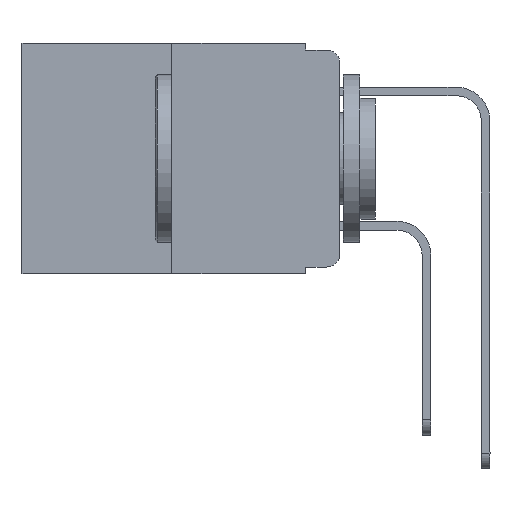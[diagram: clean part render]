
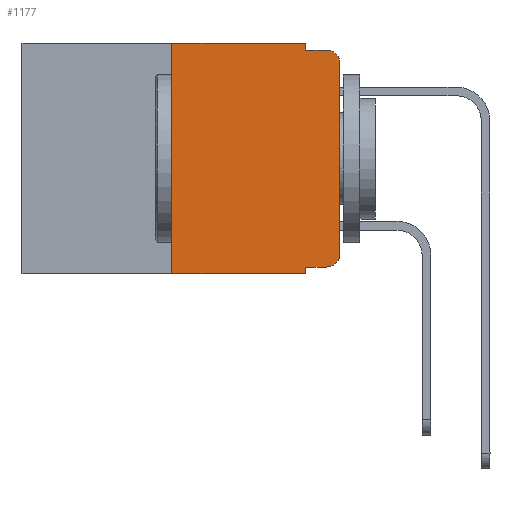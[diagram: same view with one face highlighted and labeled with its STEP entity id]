
A CAD part, left-side view. The second image highlights one B-rep face of the part: STEP entity #1177.
In plain terms, the highlighted planar face has unit normal (-1, 0, 0).
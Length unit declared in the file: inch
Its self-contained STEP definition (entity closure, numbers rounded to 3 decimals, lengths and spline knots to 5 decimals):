
#102 = EDGE_CURVE ( 'NONE', #10034, #8125, #7041, .T. ) ;
#169 = VECTOR ( 'NONE', #8905, 39.37008 ) ;
#408 = LINE ( 'NONE', #1333, #6631 ) ;
#523 = VECTOR ( 'NONE', #4066, 39.37008 ) ;
#565 = CARTESIAN_POINT ( 'NONE',  ( 0., 0.25, 0. ) ) ;
#645 = LINE ( 'NONE', #7770, #7120 ) ;
#703 = LINE ( 'NONE', #6839, #169 ) ;
#1177 = ADVANCED_FACE ( 'NONE', ( #7506 ), #9507, .F. ) ;
#1267 = CARTESIAN_POINT ( 'NONE',  ( 0., 0.02, -0.313 ) ) ;
#1333 = CARTESIAN_POINT ( 'NONE',  ( 0., 0.051, -0.333 ) ) ;
#1868 = DIRECTION ( 'NONE',  ( 0., 0., -1. ) ) ;
#2195 = AXIS2_PLACEMENT_3D ( 'NONE', #5825, #8612, #1868 ) ;
#2274 = VERTEX_POINT ( 'NONE', #9673 ) ;
#2414 = DIRECTION ( 'NONE',  ( 0., -1., 0. ) ) ;
#2418 = VECTOR ( 'NONE', #7237, 39.37008 ) ;
#2542 = CARTESIAN_POINT ( 'NONE',  ( 0., 0.25, -0.343 ) ) ;
#2949 = EDGE_CURVE ( 'NONE', #4676, #5879, #6572, .T. ) ;
#3016 = VERTEX_POINT ( 'NONE', #565 ) ;
#3075 = CARTESIAN_POINT ( 'NONE',  ( 0., 0.02, -0.333 ) ) ;
#3204 = DIRECTION ( 'NONE',  ( 0., 0., -1. ) ) ;
#3265 = ORIENTED_EDGE ( 'NONE', *, *, #8750, .T. ) ;
#3638 = DIRECTION ( 'NONE',  ( -1., 0., 0. ) ) ;
#3937 = CARTESIAN_POINT ( 'NONE',  ( 0., 0., 0. ) ) ;
#3944 = ORIENTED_EDGE ( 'NONE', *, *, #8931, .F. ) ;
#4066 = DIRECTION ( 'NONE',  ( 0., 0., 1. ) ) ;
#4118 = VERTEX_POINT ( 'NONE', #13077 ) ;
#4213 = LINE ( 'NONE', #7182, #4791 ) ;
#4479 = AXIS2_PLACEMENT_3D ( 'NONE', #11555, #5319, #10376 ) ;
#4546 = LINE ( 'NONE', #3937, #523 ) ;
#4676 = VERTEX_POINT ( 'NONE', #2542 ) ;
#4791 = VECTOR ( 'NONE', #8056, 39.37008 ) ;
#5319 = DIRECTION ( 'NONE',  ( 1., 0., 0. ) ) ;
#5446 = VECTOR ( 'NONE', #3204, 39.37008 ) ;
#5519 = VERTEX_POINT ( 'NONE', #9796 ) ;
#5686 = CARTESIAN_POINT ( 'NONE',  ( 0., 0., -0.313 ) ) ;
#5825 = CARTESIAN_POINT ( 'NONE',  ( 0., 0.02, -0.03 ) ) ;
#5879 = VERTEX_POINT ( 'NONE', #6442 ) ;
#5960 = VECTOR ( 'NONE', #2414, 39.37008 ) ;
#6274 = EDGE_LOOP ( 'NONE', ( #3265, #7491, #10293, #9197, #3944, #6538, #10992, #10276, #8016, #8421 ) ) ;
#6439 = LINE ( 'NONE', #9430, #5446 ) ;
#6442 = CARTESIAN_POINT ( 'NONE',  ( 0., 0.051, -0.343 ) ) ;
#6538 = ORIENTED_EDGE ( 'NONE', *, *, #12137, .F. ) ;
#6572 = LINE ( 'NONE', #9560, #5960 ) ;
#6631 = VECTOR ( 'NONE', #12517, 39.37008 ) ;
#6689 = EDGE_CURVE ( 'NONE', #2274, #11320, #408, .T. ) ;
#6839 = CARTESIAN_POINT ( 'NONE',  ( 0., 0.051, -0.01 ) ) ;
#6864 = EDGE_CURVE ( 'NONE', #11320, #8948, #7256, .T. ) ;
#7041 = CIRCLE ( 'NONE', #2195, 0.02 ) ;
#7092 = CARTESIAN_POINT ( 'NONE',  ( 0., 0., -0.03 ) ) ;
#7120 = VECTOR ( 'NONE', #7831, 39.37008 ) ;
#7182 = CARTESIAN_POINT ( 'NONE',  ( 0., 0.25, 0. ) ) ;
#7237 = DIRECTION ( 'NONE',  ( 0., -1., 0. ) ) ;
#7256 = CIRCLE ( 'NONE', #8959, 0.02 ) ;
#7368 = LINE ( 'NONE', #8242, #2418 ) ;
#7400 = CARTESIAN_POINT ( 'NONE',  ( 0., 0.02, -0.01 ) ) ;
#7491 = ORIENTED_EDGE ( 'NONE', *, *, #102, .T. ) ;
#7506 = FACE_OUTER_BOUND ( 'NONE', #6274, .T. ) ;
#7770 = CARTESIAN_POINT ( 'NONE',  ( 0., 0.051, 0. ) ) ;
#7831 = DIRECTION ( 'NONE',  ( 0., 0., -1. ) ) ;
#8016 = ORIENTED_EDGE ( 'NONE', *, *, #6689, .T. ) ;
#8056 = DIRECTION ( 'NONE',  ( 0., 0., 1. ) ) ;
#8125 = VERTEX_POINT ( 'NONE', #7400 ) ;
#8242 = CARTESIAN_POINT ( 'NONE',  ( 0., 0.473, 0. ) ) ;
#8421 = ORIENTED_EDGE ( 'NONE', *, *, #6864, .T. ) ;
#8612 = DIRECTION ( 'NONE',  ( -1., 0., 0. ) ) ;
#8750 = EDGE_CURVE ( 'NONE', #8948, #10034, #4546, .T. ) ;
#8905 = DIRECTION ( 'NONE',  ( 0., -1., 0. ) ) ;
#8931 = EDGE_CURVE ( 'NONE', #3016, #5519, #7368, .T. ) ;
#8948 = VERTEX_POINT ( 'NONE', #5686 ) ;
#8959 = AXIS2_PLACEMENT_3D ( 'NONE', #1267, #3638, #10663 ) ;
#9197 = ORIENTED_EDGE ( 'NONE', *, *, #12383, .F. ) ;
#9430 = CARTESIAN_POINT ( 'NONE',  ( 0., 0.051, 0. ) ) ;
#9507 = PLANE ( 'NONE',  #4479 ) ;
#9560 = CARTESIAN_POINT ( 'NONE',  ( 0., 0.473, -0.343 ) ) ;
#9673 = CARTESIAN_POINT ( 'NONE',  ( 0., 0.051, -0.333 ) ) ;
#9796 = CARTESIAN_POINT ( 'NONE',  ( 0., 0.051, 0. ) ) ;
#10034 = VERTEX_POINT ( 'NONE', #7092 ) ;
#10276 = ORIENTED_EDGE ( 'NONE', *, *, #12710, .F. ) ;
#10293 = ORIENTED_EDGE ( 'NONE', *, *, #12399, .F. ) ;
#10376 = DIRECTION ( 'NONE',  ( 0., 0., -1. ) ) ;
#10663 = DIRECTION ( 'NONE',  ( 0., 0., -1. ) ) ;
#10992 = ORIENTED_EDGE ( 'NONE', *, *, #2949, .T. ) ;
#11320 = VERTEX_POINT ( 'NONE', #3075 ) ;
#11555 = CARTESIAN_POINT ( 'NONE',  ( 0., 0.473, 0. ) ) ;
#12137 = EDGE_CURVE ( 'NONE', #4676, #3016, #4213, .T. ) ;
#12383 = EDGE_CURVE ( 'NONE', #5519, #4118, #645, .T. ) ;
#12399 = EDGE_CURVE ( 'NONE', #4118, #8125, #703, .T. ) ;
#12517 = DIRECTION ( 'NONE',  ( 0., -1., 0. ) ) ;
#12710 = EDGE_CURVE ( 'NONE', #2274, #5879, #6439, .T. ) ;
#13077 = CARTESIAN_POINT ( 'NONE',  ( 0., 0.051, -0.01 ) ) ;
